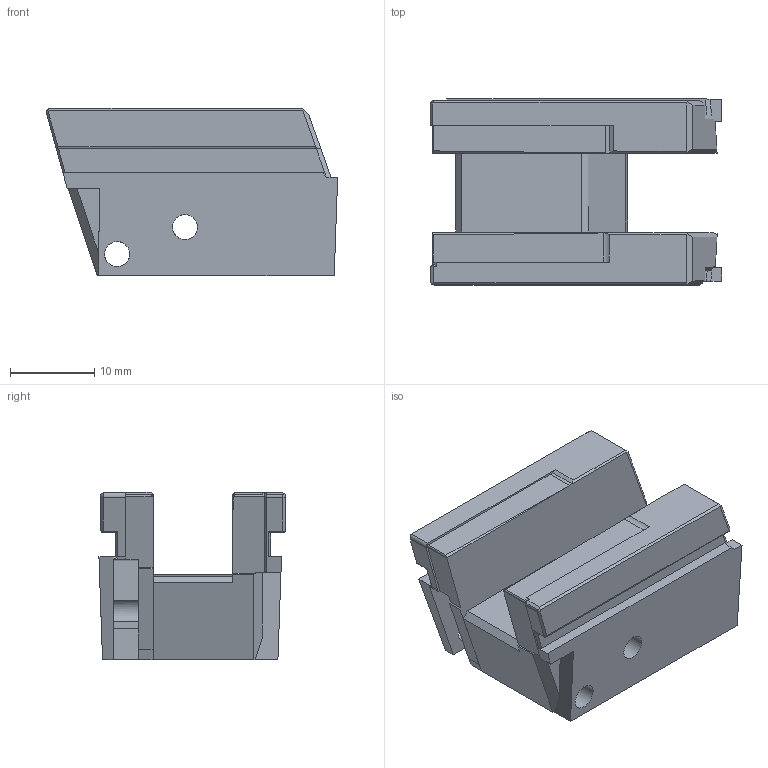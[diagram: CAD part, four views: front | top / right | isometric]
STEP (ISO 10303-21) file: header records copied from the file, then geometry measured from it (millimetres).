
FILE_DESCRIPTION(/* description */ (''),/* implementation_level */ '2;1');
FILE_NAME(/* name */ '3095 Rear Rail Block v5.step',/* time_stamp */ '2022-09-27T08:44:55-05:00',/* author */ (''),/* organization */ (''),/* preprocessor_version */ 'ST-DEVELOPER v19',/* originating_system */ 'Autodesk Translation Framework v11.7.0.108',/* authorisation */ '');
FILE_SCHEMA (('AUTOMOTIVE_DESIGN { 1 0 10303 214 3 1 1 }'));
Length unit declared in the file: millimetre
Products named in the file (1): 3095 Rear Rail Block
Bounding box: 34.65 x 22.14 x 19.87 mm (x, y, z)
Volume: 7732.9 mm3; surface area: 4575.5 mm2
Topology: 1 solids, 1 shells, 125 faces, 369 edges, 245 vertices
Faces by surface type: plane 99, cylinder 15, bspline 6, cone 5
Full cylindrical faces by diameter (mm): 3 x3
Entity records: 4452 total; most frequent: CARTESIAN_POINT 1129, ORIENTED_EDGE 738, DIRECTION 611, EDGE_CURVE 369, LINE 285, VECTOR 285, VERTEX_POINT 245, AXIS2_PLACEMENT_3D 163
